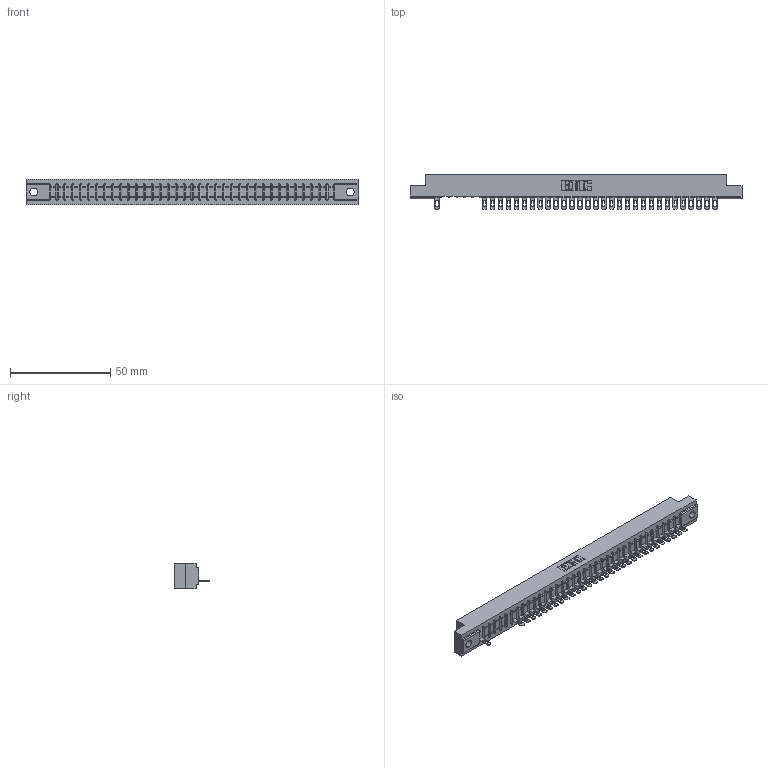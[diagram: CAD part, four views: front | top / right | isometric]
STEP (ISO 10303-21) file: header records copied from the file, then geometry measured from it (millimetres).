
FILE_DESCRIPTION (( 'STEP AP203' ), '1' );
FILE_NAME ('357-036-501-104.STEP', '2018-08-10T05:35:10', ( '' ), ( '' ), 'SwSTEP 2.0', 'SolidWorks 2016', '' );
FILE_SCHEMA (( 'CONFIG_CONTROL_DESIGN' ));
Length unit declared in the file: inch
Products named in the file (3): 307-290-002_501; 357-036-501-104; 307 Part_.156 Dia Mounting Holes
Assembly tree (32 placements, depth 2):
  357-036-501-104
    307 Part_.156 Dia Mounting Holes
    307-290-002_501  x31
Bounding box: 165.66 x 17.42 x 12.7 mm (x, y, z)
Volume: 17459.2 mm3; surface area: 20939.6 mm2
Topology: 32 solids, 32 shells, 2625 faces, 8057 edges, 5270 vertices
Faces by surface type: plane 1508, cylinder 1043, sphere 74
Entity records: 32654 total; most frequent: CARTESIAN_POINT 5533, ORIENTED_EDGE 5526, DIRECTION 5369, EDGE_CURVE 2763, VECTOR 2117, LINE 2117, VERTEX_POINT 1790, AXIS2_PLACEMENT_3D 1626
